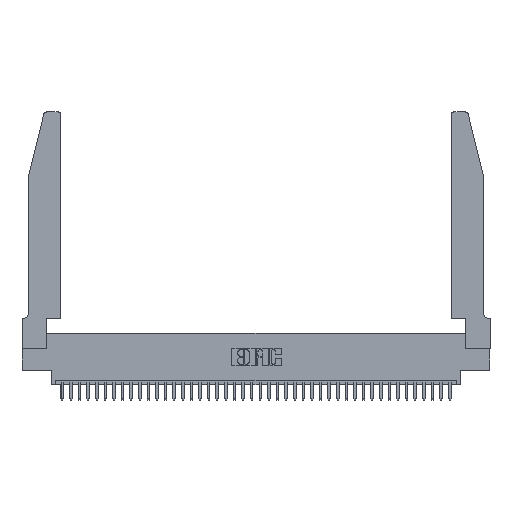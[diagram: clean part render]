
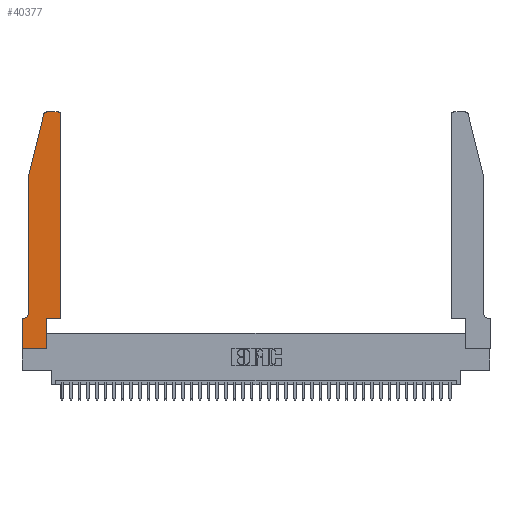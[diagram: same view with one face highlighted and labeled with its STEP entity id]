
A CAD part, top view. The second image highlights one B-rep face of the part: STEP entity #40377.
In plain terms, the highlighted planar face has unit normal (0, 0, 1).
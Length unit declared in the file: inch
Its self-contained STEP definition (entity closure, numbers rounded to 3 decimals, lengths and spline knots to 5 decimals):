
#247 = VECTOR ( 'NONE', #9127, 39.37008 ) ;
#560 = LINE ( 'NONE', #6765, #9872 ) ;
#929 = DIRECTION ( 'NONE',  ( 1., 0., 0. ) ) ;
#1314 = DIRECTION ( 'NONE',  ( 0., -1., 0. ) ) ;
#1373 = CIRCLE ( 'NONE', #31752, 0.03 ) ;
#1880 = CARTESIAN_POINT ( 'NONE',  ( 0.2865, 0.35, 0.37 ) ) ;
#2241 = ORIENTED_EDGE ( 'NONE', *, *, #27410, .T. ) ;
#3008 = DIRECTION ( 'NONE',  ( 1., 0., 0. ) ) ;
#3106 = VERTEX_POINT ( 'NONE', #6405 ) ;
#3596 = CARTESIAN_POINT ( 'NONE',  ( 0.4205, 2.75, 0.37 ) ) ;
#3844 = EDGE_CURVE ( 'NONE', #3106, #15094, #14124, .T. ) ;
#3976 = LINE ( 'NONE', #13201, #15168 ) ;
#5473 = LINE ( 'NONE', #15311, #9800 ) ;
#5680 = VECTOR ( 'NONE', #14082, 39.37008 ) ;
#6387 = CARTESIAN_POINT ( 'NONE',  ( 0., 0., 0.37 ) ) ;
#6405 = CARTESIAN_POINT ( 'NONE',  ( 0.0755, 0.42, 0.37 ) ) ;
#6577 = LINE ( 'NONE', #6387, #9521 ) ;
#6614 = LINE ( 'NONE', #27526, #247 ) ;
#6765 = CARTESIAN_POINT ( 'NONE',  ( 0., 0., 0.37 ) ) ;
#6988 = CARTESIAN_POINT ( 'NONE',  ( 0.4505, 0.35, 0.37 ) ) ;
#8192 = VERTEX_POINT ( 'NONE', #23684 ) ;
#8859 = EDGE_CURVE ( 'NONE', #32627, #25344, #6614, .T. ) ;
#9127 = DIRECTION ( 'NONE',  ( -0.239, -0.971, 0. ) ) ;
#9153 = CARTESIAN_POINT ( 'NONE',  ( 0.4505, 0.35, 0.37 ) ) ;
#9521 = VECTOR ( 'NONE', #3008, 39.37008 ) ;
#9579 = DIRECTION ( 'NONE',  ( -1., 0., 0. ) ) ;
#9800 = VECTOR ( 'NONE', #40553, 39.37008 ) ;
#9872 = VECTOR ( 'NONE', #16199, 39.37008 ) ;
#10809 = EDGE_CURVE ( 'NONE', #14073, #8192, #3976, .T. ) ;
#10915 = CARTESIAN_POINT ( 'NONE',  ( 0.4505, 0.35, 0.37 ) ) ;
#11276 = CARTESIAN_POINT ( 'NONE',  ( 0.2865, 0., 0.37 ) ) ;
#11638 = EDGE_LOOP ( 'NONE', ( #33677, #16268, #18041, #26459, #38840, #32708, #13328, #23057, #38597, #2241, #29095, #38497 ) ) ;
#11651 = DIRECTION ( 'NONE',  ( 0., 0., 1. ) ) ;
#12880 = AXIS2_PLACEMENT_3D ( 'NONE', #19392, #25978, #929 ) ;
#13201 = CARTESIAN_POINT ( 'NONE',  ( 0.2605, 2.75, 0.37 ) ) ;
#13328 = ORIENTED_EDGE ( 'NONE', *, *, #35691, .T. ) ;
#14073 = VERTEX_POINT ( 'NONE', #3596 ) ;
#14082 = DIRECTION ( 'NONE',  ( 1., 0., 0. ) ) ;
#14124 = CIRCLE ( 'NONE', #29726, 0.07 ) ;
#14851 = EDGE_CURVE ( 'NONE', #28302, #20132, #5473, .T. ) ;
#15094 = VERTEX_POINT ( 'NONE', #15240 ) ;
#15168 = VECTOR ( 'NONE', #35177, 39.37008 ) ;
#15240 = CARTESIAN_POINT ( 'NONE',  ( 0.0055, 0.35, 0.37 ) ) ;
#15311 = CARTESIAN_POINT ( 'NONE',  ( 0.2865, 0.35, 0.37 ) ) ;
#15967 = EDGE_CURVE ( 'NONE', #28989, #30638, #35806, .T. ) ;
#16015 = DIRECTION ( 'NONE',  ( -1., 0., 0. ) ) ;
#16161 = DIRECTION ( 'NONE',  ( 0., 0., -1. ) ) ;
#16199 = DIRECTION ( 'NONE',  ( 0., -1., 0. ) ) ;
#16268 = ORIENTED_EDGE ( 'NONE', *, *, #26080, .T. ) ;
#17128 = VERTEX_POINT ( 'NONE', #19574 ) ;
#18041 = ORIENTED_EDGE ( 'NONE', *, *, #8859, .T. ) ;
#18318 = LINE ( 'NONE', #22205, #37020 ) ;
#19392 = CARTESIAN_POINT ( 'NONE',  ( 0., 0.35, 0.37 ) ) ;
#19574 = CARTESIAN_POINT ( 'NONE',  ( 0., 0.35, 0.37 ) ) ;
#20132 = VERTEX_POINT ( 'NONE', #1880 ) ;
#21371 = LINE ( 'NONE', #10915, #5680 ) ;
#22142 = CARTESIAN_POINT ( 'NONE',  ( 0.284, 2.72, 0.37 ) ) ;
#22205 = CARTESIAN_POINT ( 'NONE',  ( 0.0755, 0.35, 0.37 ) ) ;
#22219 = AXIS2_PLACEMENT_3D ( 'NONE', #39790, #11651, #36529 ) ;
#22556 = EDGE_CURVE ( 'NONE', #30638, #14073, #24413, .T. ) ;
#23057 = ORIENTED_EDGE ( 'NONE', *, *, #27810, .T. ) ;
#23298 = CARTESIAN_POINT ( 'NONE',  ( 0.4505, 2.72, 0.37 ) ) ;
#23662 = CARTESIAN_POINT ( 'NONE',  ( 0.0755, 2., 0.37 ) ) ;
#23684 = CARTESIAN_POINT ( 'NONE',  ( 0.284, 2.75, 0.37 ) ) ;
#24413 = CIRCLE ( 'NONE', #22219, 0.03 ) ;
#25219 = FACE_OUTER_BOUND ( 'NONE', #11638, .T. ) ;
#25269 = DIRECTION ( 'NONE',  ( 0., 0., 1. ) ) ;
#25344 = VERTEX_POINT ( 'NONE', #37202 ) ;
#25539 = CARTESIAN_POINT ( 'NONE',  ( 0.25487, 2.72718, 0.37 ) ) ;
#25824 = PLANE ( 'NONE',  #12880 ) ;
#25978 = DIRECTION ( 'NONE',  ( 0., 0., 1. ) ) ;
#26080 = EDGE_CURVE ( 'NONE', #8192, #32627, #1373, .T. ) ;
#26459 = ORIENTED_EDGE ( 'NONE', *, *, #32957, .T. ) ;
#27410 = EDGE_CURVE ( 'NONE', #20132, #28989, #21371, .T. ) ;
#27526 = CARTESIAN_POINT ( 'NONE',  ( 0.0755, 2., 0.37 ) ) ;
#27810 = EDGE_CURVE ( 'NONE', #35984, #28302, #6577, .T. ) ;
#28302 = VERTEX_POINT ( 'NONE', #11276 ) ;
#28491 = EDGE_CURVE ( 'NONE', #15094, #17128, #18318, .T. ) ;
#28776 = VECTOR ( 'NONE', #1314, 39.37008 ) ;
#28923 = DIRECTION ( 'NONE',  ( 0., 1., 0. ) ) ;
#28989 = VERTEX_POINT ( 'NONE', #9153 ) ;
#29095 = ORIENTED_EDGE ( 'NONE', *, *, #15967, .T. ) ;
#29726 = AXIS2_PLACEMENT_3D ( 'NONE', #31418, #16161, #16015 ) ;
#29953 = CARTESIAN_POINT ( 'NONE',  ( 0., 0., 0.37 ) ) ;
#30638 = VERTEX_POINT ( 'NONE', #23298 ) ;
#31418 = CARTESIAN_POINT ( 'NONE',  ( 0.0055, 0.42, 0.37 ) ) ;
#31752 = AXIS2_PLACEMENT_3D ( 'NONE', #22142, #25269, #34514 ) ;
#32627 = VERTEX_POINT ( 'NONE', #25539 ) ;
#32708 = ORIENTED_EDGE ( 'NONE', *, *, #28491, .T. ) ;
#32957 = EDGE_CURVE ( 'NONE', #25344, #3106, #37176, .T. ) ;
#33677 = ORIENTED_EDGE ( 'NONE', *, *, #10809, .T. ) ;
#33831 = VECTOR ( 'NONE', #28923, 39.37008 ) ;
#34514 = DIRECTION ( 'NONE',  ( 1., 0., 0. ) ) ;
#35177 = DIRECTION ( 'NONE',  ( -1., 0., 0. ) ) ;
#35691 = EDGE_CURVE ( 'NONE', #17128, #35984, #560, .T. ) ;
#35806 = LINE ( 'NONE', #6988, #33831 ) ;
#35984 = VERTEX_POINT ( 'NONE', #29953 ) ;
#36529 = DIRECTION ( 'NONE',  ( 1., 0., 0. ) ) ;
#37020 = VECTOR ( 'NONE', #9579, 39.37008 ) ;
#37176 = LINE ( 'NONE', #23662, #28776 ) ;
#37202 = CARTESIAN_POINT ( 'NONE',  ( 0.0755, 2., 0.37 ) ) ;
#38497 = ORIENTED_EDGE ( 'NONE', *, *, #22556, .T. ) ;
#38597 = ORIENTED_EDGE ( 'NONE', *, *, #14851, .T. ) ;
#38840 = ORIENTED_EDGE ( 'NONE', *, *, #3844, .T. ) ;
#39790 = CARTESIAN_POINT ( 'NONE',  ( 0.4205, 2.72, 0.37 ) ) ;
#40377 = ADVANCED_FACE ( 'NONE', ( #25219 ), #25824, .T. ) ;
#40553 = DIRECTION ( 'NONE',  ( 0., 1., 0. ) ) ;
